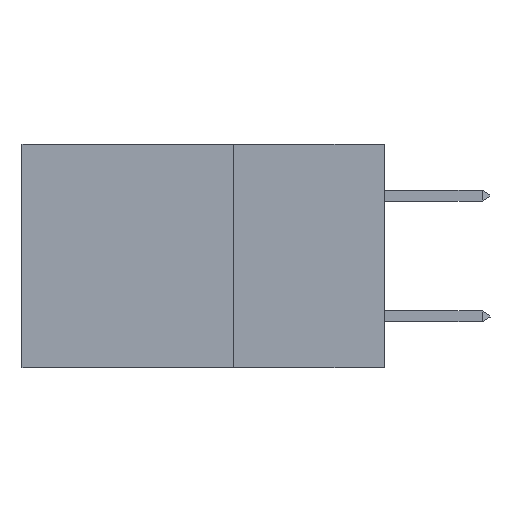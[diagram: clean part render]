
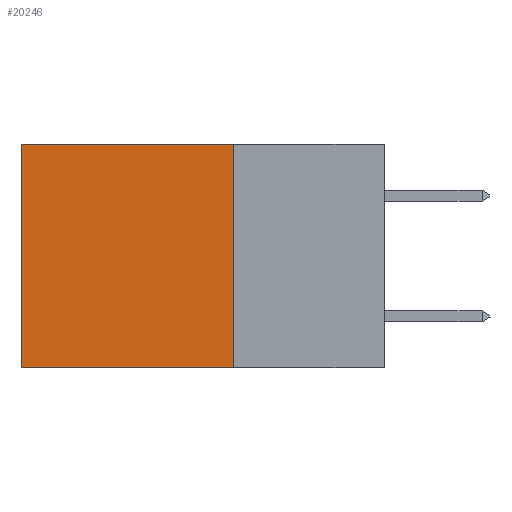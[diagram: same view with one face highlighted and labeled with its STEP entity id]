
A CAD part, left-side view. The second image highlights one B-rep face of the part: STEP entity #20246.
In plain terms, the highlighted planar face has unit normal (-1, 0, 0).
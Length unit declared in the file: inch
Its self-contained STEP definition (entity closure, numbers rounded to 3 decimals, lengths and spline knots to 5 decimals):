
#1051 = AXIS2_PLACEMENT_3D ( 'NONE', #4308, #16322, #20405 ) ;
#2426 = PLANE ( 'NONE',  #1051 ) ;
#2700 = ORIENTED_EDGE ( 'NONE', *, *, #7376, .T. ) ;
#4308 = CARTESIAN_POINT ( 'NONE',  ( 0.2875, 0.25, 0. ) ) ;
#4617 = CARTESIAN_POINT ( 'NONE',  ( 0.2875, 0.25, 0. ) ) ;
#4872 = VECTOR ( 'NONE', #20622, 39.37008 ) ;
#6450 = VERTEX_POINT ( 'NONE', #24583 ) ;
#6590 = EDGE_CURVE ( 'NONE', #6450, #15607, #16371, .T. ) ;
#7376 = EDGE_CURVE ( 'NONE', #15607, #22312, #15390, .T. ) ;
#8944 = CARTESIAN_POINT ( 'NONE',  ( 0.2875, 0.6, 0. ) ) ;
#11852 = VECTOR ( 'NONE', #12581, 39.37008 ) ;
#12581 = DIRECTION ( 'NONE',  ( 0., 0., -1. ) ) ;
#13269 = CARTESIAN_POINT ( 'NONE',  ( 0.2875, 0.6, -0.37 ) ) ;
#13892 = EDGE_LOOP ( 'NONE', ( #2700, #25103, #24864, #22102 ) ) ;
#14274 = VECTOR ( 'NONE', #22041, 39.37008 ) ;
#15390 = LINE ( 'NONE', #18722, #15717 ) ;
#15607 = VERTEX_POINT ( 'NONE', #8944 ) ;
#15717 = VECTOR ( 'NONE', #20556, 39.37008 ) ;
#16322 = DIRECTION ( 'NONE',  ( 1., 0., 0. ) ) ;
#16371 = LINE ( 'NONE', #4617, #4872 ) ;
#16507 = VERTEX_POINT ( 'NONE', #16670 ) ;
#16670 = CARTESIAN_POINT ( 'NONE',  ( 0.2875, 0.25, -0.37 ) ) ;
#17832 = LINE ( 'NONE', #18675, #11852 ) ;
#18675 = CARTESIAN_POINT ( 'NONE',  ( 0.2875, 0.25, 0. ) ) ;
#18722 = CARTESIAN_POINT ( 'NONE',  ( 0.2875, 0.6, 0. ) ) ;
#19692 = LINE ( 'NONE', #21734, #14274 ) ;
#20246 = ADVANCED_FACE ( 'NONE', ( #20532 ), #2426, .F. ) ;
#20405 = DIRECTION ( 'NONE',  ( 0., 0., -1. ) ) ;
#20532 = FACE_OUTER_BOUND ( 'NONE', #13892, .T. ) ;
#20556 = DIRECTION ( 'NONE',  ( 0., 0., -1. ) ) ;
#20622 = DIRECTION ( 'NONE',  ( 0., 1., 0. ) ) ;
#21734 = CARTESIAN_POINT ( 'NONE',  ( 0.2875, 0.25, -0.37 ) ) ;
#22041 = DIRECTION ( 'NONE',  ( 0., 1., 0. ) ) ;
#22102 = ORIENTED_EDGE ( 'NONE', *, *, #6590, .T. ) ;
#22312 = VERTEX_POINT ( 'NONE', #13269 ) ;
#24574 = EDGE_CURVE ( 'NONE', #6450, #16507, #17832, .T. ) ;
#24583 = CARTESIAN_POINT ( 'NONE',  ( 0.2875, 0.25, 0. ) ) ;
#24864 = ORIENTED_EDGE ( 'NONE', *, *, #24574, .F. ) ;
#25103 = ORIENTED_EDGE ( 'NONE', *, *, #25665, .F. ) ;
#25665 = EDGE_CURVE ( 'NONE', #16507, #22312, #19692, .T. ) ;
